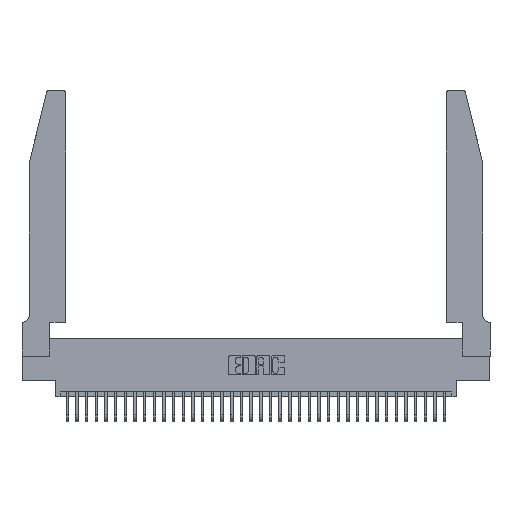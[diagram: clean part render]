
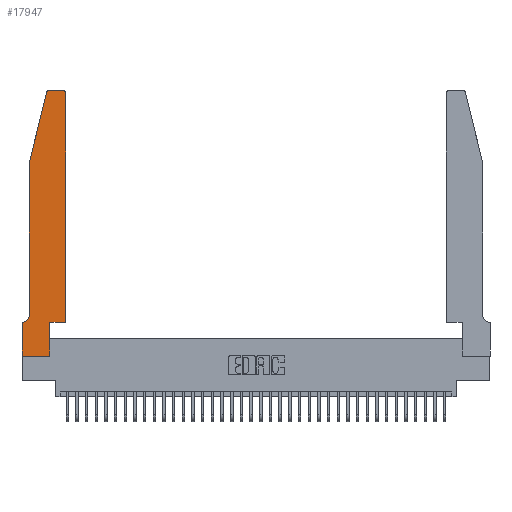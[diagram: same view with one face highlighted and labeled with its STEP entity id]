
A CAD part, top view. The second image highlights one B-rep face of the part: STEP entity #17947.
In plain terms, the highlighted planar face has unit normal (0, 0, 1).
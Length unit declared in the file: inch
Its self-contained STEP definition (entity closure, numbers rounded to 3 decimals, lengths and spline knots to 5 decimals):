
#24 = VERTEX_POINT ( 'NONE', #3588 ) ;
#560 = CARTESIAN_POINT ( 'NONE',  ( 0.25487, 2.72718, 0.37 ) ) ;
#791 = LINE ( 'NONE', #38048, #25454 ) ;
#1469 = VECTOR ( 'NONE', #17944, 39.37008 ) ;
#1599 = ORIENTED_EDGE ( 'NONE', *, *, #7758, .T. ) ;
#2123 = AXIS2_PLACEMENT_3D ( 'NONE', #15376, #35829, #18302 ) ;
#2329 = ORIENTED_EDGE ( 'NONE', *, *, #27461, .T. ) ;
#2338 = CARTESIAN_POINT ( 'NONE',  ( 0.0055, 0.42, 0.37 ) ) ;
#2737 = CIRCLE ( 'NONE', #2123, 0.03 ) ;
#3567 = CARTESIAN_POINT ( 'NONE',  ( 0.4505, 0.35, 0.37 ) ) ;
#3588 = CARTESIAN_POINT ( 'NONE',  ( 0.2865, 0.35, 0.37 ) ) ;
#4197 = DIRECTION ( 'NONE',  ( 0., -1., 0. ) ) ;
#4357 = EDGE_CURVE ( 'NONE', #37479, #13511, #32556, .T. ) ;
#4471 = CARTESIAN_POINT ( 'NONE',  ( 0.0755, 2., 0.37 ) ) ;
#4492 = FACE_OUTER_BOUND ( 'NONE', #16428, .T. ) ;
#5356 = DIRECTION ( 'NONE',  ( -1., 0., 0. ) ) ;
#6326 = ORIENTED_EDGE ( 'NONE', *, *, #25473, .T. ) ;
#6439 = CARTESIAN_POINT ( 'NONE',  ( 0.0755, 0.42, 0.37 ) ) ;
#6462 = VERTEX_POINT ( 'NONE', #27941 ) ;
#6931 = VERTEX_POINT ( 'NONE', #15481 ) ;
#7201 = CARTESIAN_POINT ( 'NONE',  ( 0., 0.35, 0.37 ) ) ;
#7572 = CARTESIAN_POINT ( 'NONE',  ( 0.0755, 2., 0.37 ) ) ;
#7758 = EDGE_CURVE ( 'NONE', #6931, #24944, #19943, .T. ) ;
#8489 = PLANE ( 'NONE',  #21838 ) ;
#8891 = DIRECTION ( 'NONE',  ( -1., 0., 0. ) ) ;
#9040 = DIRECTION ( 'NONE',  ( 0., 1., 0. ) ) ;
#9562 = VERTEX_POINT ( 'NONE', #6439 ) ;
#11340 = CARTESIAN_POINT ( 'NONE',  ( 0., 0., 0.37 ) ) ;
#11449 = ORIENTED_EDGE ( 'NONE', *, *, #15895, .T. ) ;
#11505 = DIRECTION ( 'NONE',  ( 0., 0., 1. ) ) ;
#11862 = AXIS2_PLACEMENT_3D ( 'NONE', #2338, #23119, #5356 ) ;
#12385 = AXIS2_PLACEMENT_3D ( 'NONE', #33733, #16210, #36638 ) ;
#12533 = ORIENTED_EDGE ( 'NONE', *, *, #22796, .T. ) ;
#12940 = VERTEX_POINT ( 'NONE', #16001 ) ;
#13156 = CARTESIAN_POINT ( 'NONE',  ( 0.2605, 2.75, 0.37 ) ) ;
#13377 = LINE ( 'NONE', #7572, #28068 ) ;
#13460 = EDGE_CURVE ( 'NONE', #24, #12940, #30667, .T. ) ;
#13511 = VERTEX_POINT ( 'NONE', #30422 ) ;
#14771 = DIRECTION ( 'NONE',  ( 0., 1., 0. ) ) ;
#15376 = CARTESIAN_POINT ( 'NONE',  ( 0.4205, 2.72, 0.37 ) ) ;
#15481 = CARTESIAN_POINT ( 'NONE',  ( 0.284, 2.75, 0.37 ) ) ;
#15895 = EDGE_CURVE ( 'NONE', #25601, #6931, #36021, .T. ) ;
#16001 = CARTESIAN_POINT ( 'NONE',  ( 0.4505, 0.35, 0.37 ) ) ;
#16210 = DIRECTION ( 'NONE',  ( 0., 0., 1. ) ) ;
#16290 = LINE ( 'NONE', #11340, #31879 ) ;
#16428 = EDGE_LOOP ( 'NONE', ( #11449, #1599, #24431, #6326, #2329, #25485, #25140, #12533, #31965, #19832, #18805, #30790 ) ) ;
#16951 = EDGE_CURVE ( 'NONE', #6462, #25601, #2737, .T. ) ;
#17348 = CARTESIAN_POINT ( 'NONE',  ( 0., 0.35, 0.37 ) ) ;
#17716 = LINE ( 'NONE', #26775, #18637 ) ;
#17817 = CARTESIAN_POINT ( 'NONE',  ( 0.0755, 2., 0.37 ) ) ;
#17894 = VECTOR ( 'NONE', #4197, 39.37008 ) ;
#17944 = DIRECTION ( 'NONE',  ( -0.239, -0.971, 0. ) ) ;
#17947 = ADVANCED_FACE ( 'NONE', ( #4492 ), #8489, .T. ) ;
#18302 = DIRECTION ( 'NONE',  ( 1., 0., 0. ) ) ;
#18637 = VECTOR ( 'NONE', #9040, 39.37008 ) ;
#18805 = ORIENTED_EDGE ( 'NONE', *, *, #22045, .T. ) ;
#19018 = CARTESIAN_POINT ( 'NONE',  ( 0., 0., 0.37 ) ) ;
#19079 = DIRECTION ( 'NONE',  ( -1., 0., 0. ) ) ;
#19832 = ORIENTED_EDGE ( 'NONE', *, *, #13460, .T. ) ;
#19943 = CIRCLE ( 'NONE', #12385, 0.03 ) ;
#20651 = VERTEX_POINT ( 'NONE', #4471 ) ;
#21838 = AXIS2_PLACEMENT_3D ( 'NONE', #17348, #11505, #32083 ) ;
#22000 = VECTOR ( 'NONE', #36027, 39.37008 ) ;
#22045 = EDGE_CURVE ( 'NONE', #12940, #6462, #17716, .T. ) ;
#22142 = VECTOR ( 'NONE', #14771, 39.37008 ) ;
#22357 = DIRECTION ( 'NONE',  ( 0., -1., 0. ) ) ;
#22796 = EDGE_CURVE ( 'NONE', #13511, #26106, #16290, .T. ) ;
#23119 = DIRECTION ( 'NONE',  ( 0., 0., -1. ) ) ;
#24431 = ORIENTED_EDGE ( 'NONE', *, *, #31764, .T. ) ;
#24793 = CIRCLE ( 'NONE', #11862, 0.07 ) ;
#24944 = VERTEX_POINT ( 'NONE', #560 ) ;
#25140 = ORIENTED_EDGE ( 'NONE', *, *, #4357, .T. ) ;
#25454 = VECTOR ( 'NONE', #8891, 39.37008 ) ;
#25473 = EDGE_CURVE ( 'NONE', #20651, #9562, #13377, .T. ) ;
#25485 = ORIENTED_EDGE ( 'NONE', *, *, #36595, .T. ) ;
#25601 = VERTEX_POINT ( 'NONE', #28747 ) ;
#26106 = VERTEX_POINT ( 'NONE', #37334 ) ;
#26775 = CARTESIAN_POINT ( 'NONE',  ( 0.4505, 0.35, 0.37 ) ) ;
#27461 = EDGE_CURVE ( 'NONE', #9562, #36167, #24793, .T. ) ;
#27549 = CARTESIAN_POINT ( 'NONE',  ( 0.0055, 0.35, 0.37 ) ) ;
#27941 = CARTESIAN_POINT ( 'NONE',  ( 0.4505, 2.72, 0.37 ) ) ;
#28068 = VECTOR ( 'NONE', #22357, 39.37008 ) ;
#28292 = VECTOR ( 'NONE', #19079, 39.37008 ) ;
#28747 = CARTESIAN_POINT ( 'NONE',  ( 0.4205, 2.75, 0.37 ) ) ;
#30422 = CARTESIAN_POINT ( 'NONE',  ( 0., 0., 0.37 ) ) ;
#30667 = LINE ( 'NONE', #3567, #22000 ) ;
#30790 = ORIENTED_EDGE ( 'NONE', *, *, #16951, .T. ) ;
#31764 = EDGE_CURVE ( 'NONE', #24944, #20651, #33851, .T. ) ;
#31879 = VECTOR ( 'NONE', #31925, 39.37008 ) ;
#31925 = DIRECTION ( 'NONE',  ( 1., 0., 0. ) ) ;
#31965 = ORIENTED_EDGE ( 'NONE', *, *, #37797, .T. ) ;
#32083 = DIRECTION ( 'NONE',  ( 1., 0., 0. ) ) ;
#32556 = LINE ( 'NONE', #19018, #17894 ) ;
#33733 = CARTESIAN_POINT ( 'NONE',  ( 0.284, 2.72, 0.37 ) ) ;
#33851 = LINE ( 'NONE', #17817, #1469 ) ;
#35234 = CARTESIAN_POINT ( 'NONE',  ( 0.2865, 0.35, 0.37 ) ) ;
#35829 = DIRECTION ( 'NONE',  ( 0., 0., 1. ) ) ;
#36021 = LINE ( 'NONE', #13156, #28292 ) ;
#36027 = DIRECTION ( 'NONE',  ( 1., 0., 0. ) ) ;
#36167 = VERTEX_POINT ( 'NONE', #27549 ) ;
#36595 = EDGE_CURVE ( 'NONE', #36167, #37479, #791, .T. ) ;
#36638 = DIRECTION ( 'NONE',  ( 1., 0., 0. ) ) ;
#37334 = CARTESIAN_POINT ( 'NONE',  ( 0.2865, 0., 0.37 ) ) ;
#37479 = VERTEX_POINT ( 'NONE', #7201 ) ;
#37625 = LINE ( 'NONE', #35234, #22142 ) ;
#37797 = EDGE_CURVE ( 'NONE', #26106, #24, #37625, .T. ) ;
#38048 = CARTESIAN_POINT ( 'NONE',  ( 0.0755, 0.35, 0.37 ) ) ;
